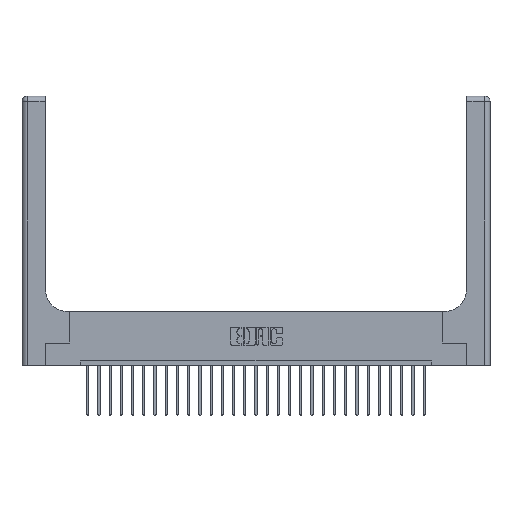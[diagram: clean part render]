
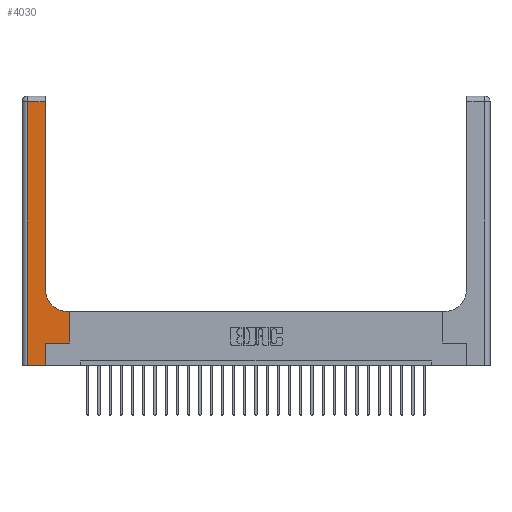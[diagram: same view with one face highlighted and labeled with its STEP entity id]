
A CAD part, top view. The second image highlights one B-rep face of the part: STEP entity #4030.
In plain terms, the highlighted planar face has unit normal (0, 0, 1).
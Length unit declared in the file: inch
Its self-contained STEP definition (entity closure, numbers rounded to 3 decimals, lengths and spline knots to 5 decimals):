
#689 = DIRECTION ( 'NONE',  ( -1., 0., 0. ) ) ;
#1226 = VERTEX_POINT ( 'NONE', #16532 ) ;
#1312 = EDGE_CURVE ( 'NONE', #3821, #9793, #15586, .T. ) ;
#1801 = DIRECTION ( 'NONE',  ( 0., 1., 0. ) ) ;
#2002 = DIRECTION ( 'NONE',  ( -1., 0., 0. ) ) ;
#2450 = DIRECTION ( 'NONE',  ( 1., 0., 0. ) ) ;
#2498 = ORIENTED_EDGE ( 'NONE', *, *, #8083, .T. ) ;
#2966 = CARTESIAN_POINT ( 'NONE',  ( 0.265, 0., 0.37 ) ) ;
#3049 = VECTOR ( 'NONE', #1801, 39.37008 ) ;
#3821 = VERTEX_POINT ( 'NONE', #2966 ) ;
#4003 = VECTOR ( 'NONE', #25337, 39.37008 ) ;
#4030 = ADVANCED_FACE ( 'NONE', ( #11497 ), #5992, .F. ) ;
#4776 = DIRECTION ( 'NONE',  ( 1., 0., 0. ) ) ;
#4931 = EDGE_CURVE ( 'NONE', #16347, #1226, #16620, .T. ) ;
#5409 = EDGE_LOOP ( 'NONE', ( #22473, #16059, #19400, #20839, #7354, #9858, #2498, #24646, #14960 ) ) ;
#5500 = LINE ( 'NONE', #21514, #12420 ) ;
#5855 = EDGE_CURVE ( 'NONE', #24853, #16862, #6799, .T. ) ;
#5930 = LINE ( 'NONE', #21672, #11634 ) ;
#5992 = PLANE ( 'NONE',  #7648 ) ;
#6466 = CARTESIAN_POINT ( 'NONE',  ( 0.528, 0.25, 0.37 ) ) ;
#6799 = LINE ( 'NONE', #20953, #17950 ) ;
#7354 = ORIENTED_EDGE ( 'NONE', *, *, #1312, .T. ) ;
#7648 = AXIS2_PLACEMENT_3D ( 'NONE', #14126, #22267, #2002 ) ;
#7756 = CARTESIAN_POINT ( 'NONE',  ( 0.06, 2.94, 0.37 ) ) ;
#8083 = EDGE_CURVE ( 'NONE', #12154, #24697, #5500, .T. ) ;
#8313 = DIRECTION ( 'NONE',  ( 0., -1., 0. ) ) ;
#8515 = CARTESIAN_POINT ( 'NONE',  ( 0.06, 0., 0.37 ) ) ;
#9095 = EDGE_CURVE ( 'NONE', #9973, #3821, #5930, .T. ) ;
#9119 = CARTESIAN_POINT ( 'NONE',  ( 0.528, 0.6, 0.37 ) ) ;
#9765 = VECTOR ( 'NONE', #19314, 39.37008 ) ;
#9793 = VERTEX_POINT ( 'NONE', #19629 ) ;
#9858 = ORIENTED_EDGE ( 'NONE', *, *, #25809, .T. ) ;
#9973 = VERTEX_POINT ( 'NONE', #8515 ) ;
#10897 = CARTESIAN_POINT ( 'NONE',  ( 0.26, 0.6, 0.37 ) ) ;
#11497 = FACE_OUTER_BOUND ( 'NONE', #5409, .T. ) ;
#11563 = LINE ( 'NONE', #19713, #3049 ) ;
#11634 = VECTOR ( 'NONE', #11682, 39.37008 ) ;
#11682 = DIRECTION ( 'NONE',  ( 1., 0., 0. ) ) ;
#11734 = EDGE_CURVE ( 'NONE', #24697, #16347, #14882, .T. ) ;
#12154 = VERTEX_POINT ( 'NONE', #6466 ) ;
#12317 = LINE ( 'NONE', #20464, #25253 ) ;
#12420 = VECTOR ( 'NONE', #23249, 39.37008 ) ;
#14126 = CARTESIAN_POINT ( 'NONE',  ( 0., 3., 0.37 ) ) ;
#14882 = LINE ( 'NONE', #10897, #9765 ) ;
#14960 = ORIENTED_EDGE ( 'NONE', *, *, #4931, .T. ) ;
#15062 = CARTESIAN_POINT ( 'NONE',  ( 0.265, 0., 0.37 ) ) ;
#15309 = CARTESIAN_POINT ( 'NONE',  ( 0.265, 0.25, 0.37 ) ) ;
#15586 = LINE ( 'NONE', #15062, #4003 ) ;
#15911 = EDGE_CURVE ( 'NONE', #1226, #24853, #11563, .T. ) ;
#16059 = ORIENTED_EDGE ( 'NONE', *, *, #5855, .T. ) ;
#16347 = VERTEX_POINT ( 'NONE', #17900 ) ;
#16453 = DIRECTION ( 'NONE',  ( 0., 0., -1. ) ) ;
#16486 = VECTOR ( 'NONE', #4776, 39.37008 ) ;
#16532 = CARTESIAN_POINT ( 'NONE',  ( 0.26, 0.85, 0.37 ) ) ;
#16620 = CIRCLE ( 'NONE', #18764, 0.25 ) ;
#16862 = VERTEX_POINT ( 'NONE', #7756 ) ;
#17194 = LINE ( 'NONE', #15309, #16486 ) ;
#17719 = EDGE_CURVE ( 'NONE', #16862, #9973, #12317, .T. ) ;
#17900 = CARTESIAN_POINT ( 'NONE',  ( 0.51, 0.6, 0.37 ) ) ;
#17950 = VECTOR ( 'NONE', #689, 39.37008 ) ;
#18764 = AXIS2_PLACEMENT_3D ( 'NONE', #20719, #16453, #2450 ) ;
#19314 = DIRECTION ( 'NONE',  ( -1., 0., 0. ) ) ;
#19400 = ORIENTED_EDGE ( 'NONE', *, *, #17719, .T. ) ;
#19629 = CARTESIAN_POINT ( 'NONE',  ( 0.265, 0.25, 0.37 ) ) ;
#19713 = CARTESIAN_POINT ( 'NONE',  ( 0.26, 3., 0.37 ) ) ;
#20464 = CARTESIAN_POINT ( 'NONE',  ( 0.06, 3., 0.37 ) ) ;
#20719 = CARTESIAN_POINT ( 'NONE',  ( 0.51, 0.85, 0.37 ) ) ;
#20839 = ORIENTED_EDGE ( 'NONE', *, *, #9095, .T. ) ;
#20953 = CARTESIAN_POINT ( 'NONE',  ( 0., 2.94, 0.37 ) ) ;
#21514 = CARTESIAN_POINT ( 'NONE',  ( 0.528, 0.25, 0.37 ) ) ;
#21672 = CARTESIAN_POINT ( 'NONE',  ( 0., 0., 0.37 ) ) ;
#22267 = DIRECTION ( 'NONE',  ( 0., 0., -1. ) ) ;
#22473 = ORIENTED_EDGE ( 'NONE', *, *, #15911, .T. ) ;
#23249 = DIRECTION ( 'NONE',  ( 0., 1., 0. ) ) ;
#23387 = CARTESIAN_POINT ( 'NONE',  ( 0.26, 2.94, 0.37 ) ) ;
#24646 = ORIENTED_EDGE ( 'NONE', *, *, #11734, .T. ) ;
#24697 = VERTEX_POINT ( 'NONE', #9119 ) ;
#24853 = VERTEX_POINT ( 'NONE', #23387 ) ;
#25253 = VECTOR ( 'NONE', #8313, 39.37008 ) ;
#25337 = DIRECTION ( 'NONE',  ( 0., 1., 0. ) ) ;
#25809 = EDGE_CURVE ( 'NONE', #9793, #12154, #17194, .T. ) ;
